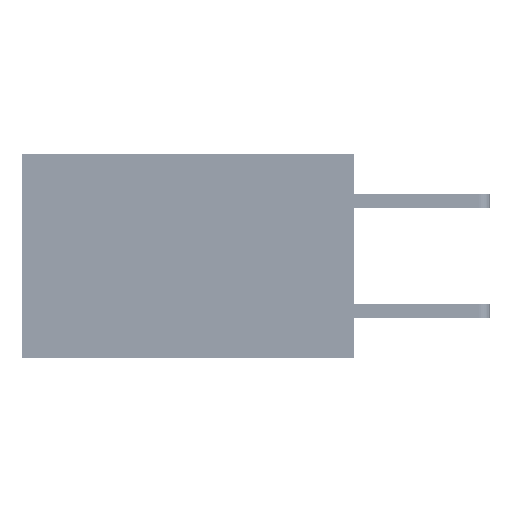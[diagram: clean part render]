
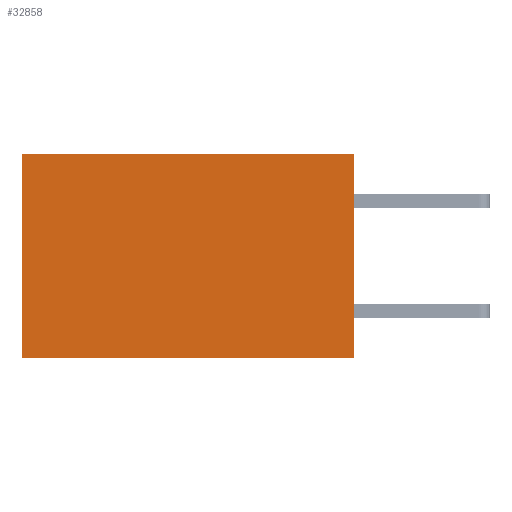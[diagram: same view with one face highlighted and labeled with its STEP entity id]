
A CAD part, left-side view. The second image highlights one B-rep face of the part: STEP entity #32858.
In plain terms, the highlighted planar face has unit normal (-1, 0, 0).
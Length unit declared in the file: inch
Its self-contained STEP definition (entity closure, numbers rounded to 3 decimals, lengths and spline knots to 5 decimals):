
#165 = PLANE ( 'NONE',  #27025 ) ;
#3446 = EDGE_CURVE ( 'NONE', #24636, #44488, #33224, .T. ) ;
#5080 = EDGE_LOOP ( 'NONE', ( #13151, #31182, #19467, #37929 ) ) ;
#7111 = VECTOR ( 'NONE', #23754, 39.37008 ) ;
#10829 = DIRECTION ( 'NONE',  ( 1., 0., 0. ) ) ;
#11796 = CARTESIAN_POINT ( 'NONE',  ( 0.2875, 0.6, 0. ) ) ;
#12492 = CARTESIAN_POINT ( 'NONE',  ( 0.2875, 0.6, -0.37 ) ) ;
#12585 = LINE ( 'NONE', #26936, #7111 ) ;
#13151 = ORIENTED_EDGE ( 'NONE', *, *, #3446, .T. ) ;
#14447 = CARTESIAN_POINT ( 'NONE',  ( 0.2875, 0., 0. ) ) ;
#15425 = DIRECTION ( 'NONE',  ( 0., 0., -1. ) ) ;
#15546 = CARTESIAN_POINT ( 'NONE',  ( 0.2875, 0., 0. ) ) ;
#15588 = CARTESIAN_POINT ( 'NONE',  ( 0.2875, 0., 0. ) ) ;
#16109 = CARTESIAN_POINT ( 'NONE',  ( 0.2875, 0., -0.37 ) ) ;
#18338 = VECTOR ( 'NONE', #37085, 39.37008 ) ;
#18386 = EDGE_CURVE ( 'NONE', #42526, #29620, #42664, .T. ) ;
#19467 = ORIENTED_EDGE ( 'NONE', *, *, #18386, .F. ) ;
#21457 = VECTOR ( 'NONE', #25834, 39.37008 ) ;
#23754 = DIRECTION ( 'NONE',  ( 0., 1., 0. ) ) ;
#24636 = VERTEX_POINT ( 'NONE', #38564 ) ;
#25834 = DIRECTION ( 'NONE',  ( 0., 0., -1. ) ) ;
#26936 = CARTESIAN_POINT ( 'NONE',  ( 0.2875, 0., -0.37 ) ) ;
#27016 = CARTESIAN_POINT ( 'NONE',  ( 0.2875, 0., 0. ) ) ;
#27025 = AXIS2_PLACEMENT_3D ( 'NONE', #14447, #10829, #42241 ) ;
#29194 = LINE ( 'NONE', #27016, #18338 ) ;
#29620 = VERTEX_POINT ( 'NONE', #16109 ) ;
#31182 = ORIENTED_EDGE ( 'NONE', *, *, #40790, .F. ) ;
#32858 = ADVANCED_FACE ( 'NONE', ( #43976 ), #165, .F. ) ;
#33224 = LINE ( 'NONE', #11796, #39780 ) ;
#33804 = EDGE_CURVE ( 'NONE', #42526, #24636, #29194, .T. ) ;
#37085 = DIRECTION ( 'NONE',  ( 0., 1., 0. ) ) ;
#37929 = ORIENTED_EDGE ( 'NONE', *, *, #33804, .T. ) ;
#38564 = CARTESIAN_POINT ( 'NONE',  ( 0.2875, 0.6, 0. ) ) ;
#39780 = VECTOR ( 'NONE', #15425, 39.37008 ) ;
#40790 = EDGE_CURVE ( 'NONE', #29620, #44488, #12585, .T. ) ;
#42241 = DIRECTION ( 'NONE',  ( 0., 0., -1. ) ) ;
#42526 = VERTEX_POINT ( 'NONE', #15588 ) ;
#42664 = LINE ( 'NONE', #15546, #21457 ) ;
#43976 = FACE_OUTER_BOUND ( 'NONE', #5080, .T. ) ;
#44488 = VERTEX_POINT ( 'NONE', #12492 ) ;
